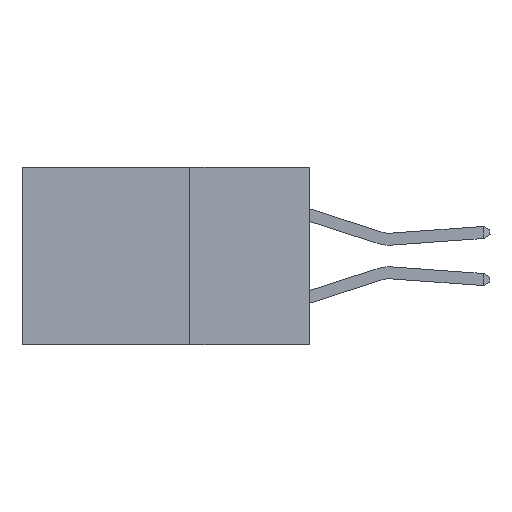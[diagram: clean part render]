
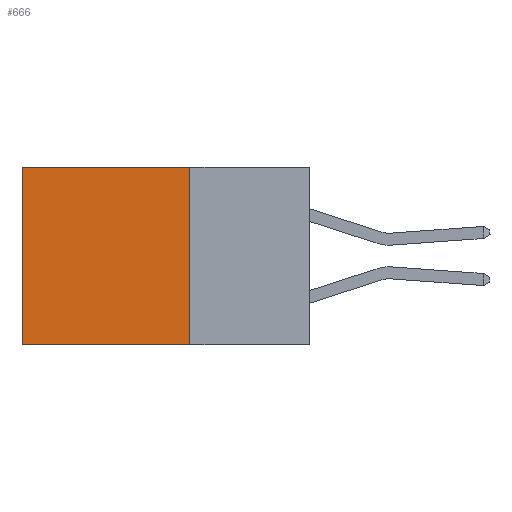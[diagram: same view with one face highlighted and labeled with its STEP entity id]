
A CAD part, left-side view. The second image highlights one B-rep face of the part: STEP entity #666.
In plain terms, the highlighted planar face has unit normal (-1, 0, 0).
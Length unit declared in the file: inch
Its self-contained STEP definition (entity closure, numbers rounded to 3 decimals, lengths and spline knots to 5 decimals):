
#666 = ADVANCED_FACE ( 'NONE', ( #10472 ), #17596, .F. ) ;
#711 = DIRECTION ( 'NONE',  ( 0., 1., 0. ) ) ;
#984 = EDGE_CURVE ( 'NONE', #20135, #8980, #17565, .T. ) ;
#1425 = ORIENTED_EDGE ( 'NONE', *, *, #984, .T. ) ;
#1614 = CARTESIAN_POINT ( 'NONE',  ( 0.2615, 0.25, -0.37 ) ) ;
#1943 = VECTOR ( 'NONE', #22579, 39.37008 ) ;
#1978 = VECTOR ( 'NONE', #21290, 39.37008 ) ;
#3671 = CARTESIAN_POINT ( 'NONE',  ( 0.2615, 0.25, 0. ) ) ;
#4677 = LINE ( 'NONE', #10045, #6009 ) ;
#6009 = VECTOR ( 'NONE', #711, 39.37008 ) ;
#7302 = VERTEX_POINT ( 'NONE', #17134 ) ;
#8353 = CARTESIAN_POINT ( 'NONE',  ( 0.2615, 0.25, -0.37 ) ) ;
#8650 = CARTESIAN_POINT ( 'NONE',  ( 0.2615, 0.25, 0. ) ) ;
#8980 = VERTEX_POINT ( 'NONE', #21897 ) ;
#10045 = CARTESIAN_POINT ( 'NONE',  ( 0.2615, 0.25, -0.37 ) ) ;
#10099 = CARTESIAN_POINT ( 'NONE',  ( 0.2615, 0.6, -0.37 ) ) ;
#10156 = AXIS2_PLACEMENT_3D ( 'NONE', #1614, #19456, #22950 ) ;
#10179 = EDGE_LOOP ( 'NONE', ( #22201, #13857, #14256, #1425 ) ) ;
#10472 = FACE_OUTER_BOUND ( 'NONE', #10179, .T. ) ;
#11855 = LINE ( 'NONE', #8353, #1943 ) ;
#13046 = VECTOR ( 'NONE', #20709, 39.37008 ) ;
#13857 = ORIENTED_EDGE ( 'NONE', *, *, #20480, .F. ) ;
#14256 = ORIENTED_EDGE ( 'NONE', *, *, #21636, .F. ) ;
#17134 = CARTESIAN_POINT ( 'NONE',  ( 0.2615, 0.25, -0.37 ) ) ;
#17565 = LINE ( 'NONE', #3671, #1978 ) ;
#17596 = PLANE ( 'NONE',  #10156 ) ;
#17679 = VERTEX_POINT ( 'NONE', #19328 ) ;
#18967 = LINE ( 'NONE', #10099, #13046 ) ;
#19328 = CARTESIAN_POINT ( 'NONE',  ( 0.2615, 0.6, -0.37 ) ) ;
#19423 = EDGE_CURVE ( 'NONE', #8980, #17679, #18967, .T. ) ;
#19456 = DIRECTION ( 'NONE',  ( 1., 0., 0. ) ) ;
#20135 = VERTEX_POINT ( 'NONE', #8650 ) ;
#20480 = EDGE_CURVE ( 'NONE', #7302, #17679, #4677, .T. ) ;
#20709 = DIRECTION ( 'NONE',  ( 0., 0., -1. ) ) ;
#21290 = DIRECTION ( 'NONE',  ( 0., 1., 0. ) ) ;
#21636 = EDGE_CURVE ( 'NONE', #20135, #7302, #11855, .T. ) ;
#21897 = CARTESIAN_POINT ( 'NONE',  ( 0.2615, 0.6, 0. ) ) ;
#22201 = ORIENTED_EDGE ( 'NONE', *, *, #19423, .T. ) ;
#22579 = DIRECTION ( 'NONE',  ( 0., 0., -1. ) ) ;
#22950 = DIRECTION ( 'NONE',  ( 0., 0., -1. ) ) ;
